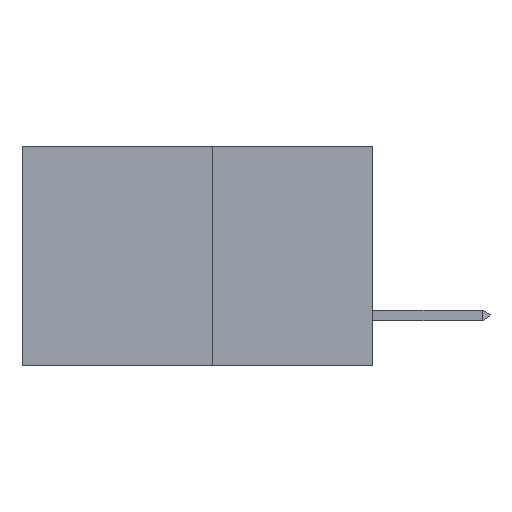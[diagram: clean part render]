
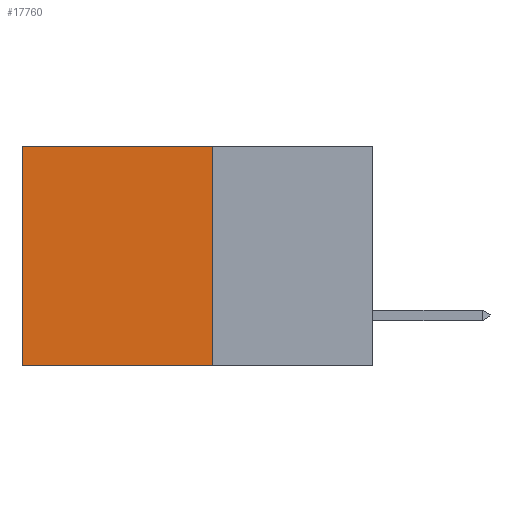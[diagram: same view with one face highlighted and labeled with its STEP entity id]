
A CAD part, left-side view. The second image highlights one B-rep face of the part: STEP entity #17760.
In plain terms, the highlighted planar face has unit normal (-1, 0, 0).
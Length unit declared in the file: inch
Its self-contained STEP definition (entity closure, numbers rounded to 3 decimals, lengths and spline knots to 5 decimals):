
#334 = CARTESIAN_POINT ( 'NONE',  ( 0.277, 0.27, -0.37 ) ) ;
#460 = VERTEX_POINT ( 'NONE', #13434 ) ;
#634 = DIRECTION ( 'NONE',  ( 0., 0., -1. ) ) ;
#1113 = CARTESIAN_POINT ( 'NONE',  ( 0.277, 0.27, 0. ) ) ;
#1631 = PLANE ( 'NONE',  #6819 ) ;
#2547 = VECTOR ( 'NONE', #6142, 39.37008 ) ;
#2607 = VECTOR ( 'NONE', #12795, 39.37008 ) ;
#2858 = CARTESIAN_POINT ( 'NONE',  ( 0.277, 0.59, -0.37 ) ) ;
#2998 = VERTEX_POINT ( 'NONE', #334 ) ;
#3637 = CARTESIAN_POINT ( 'NONE',  ( 0.277, 0.59, 0. ) ) ;
#3745 = EDGE_CURVE ( 'NONE', #14282, #460, #6698, .T. ) ;
#3871 = ORIENTED_EDGE ( 'NONE', *, *, #11626, .F. ) ;
#4233 = ORIENTED_EDGE ( 'NONE', *, *, #17497, .T. ) ;
#5212 = DIRECTION ( 'NONE',  ( 1., 0., 0. ) ) ;
#5300 = VECTOR ( 'NONE', #15342, 39.37008 ) ;
#6118 = VECTOR ( 'NONE', #634, 39.37008 ) ;
#6142 = DIRECTION ( 'NONE',  ( 0., 1., 0. ) ) ;
#6681 = LINE ( 'NONE', #9421, #6118 ) ;
#6698 = LINE ( 'NONE', #2858, #2607 ) ;
#6819 = AXIS2_PLACEMENT_3D ( 'NONE', #14176, #5212, #17722 ) ;
#7753 = LINE ( 'NONE', #15107, #2547 ) ;
#7921 = FACE_OUTER_BOUND ( 'NONE', #13401, .T. ) ;
#8155 = EDGE_CURVE ( 'NONE', #2998, #460, #7753, .T. ) ;
#9421 = CARTESIAN_POINT ( 'NONE',  ( 0.277, 0.27, -0.37 ) ) ;
#9918 = CARTESIAN_POINT ( 'NONE',  ( 0.277, 0.27, 0. ) ) ;
#11232 = ORIENTED_EDGE ( 'NONE', *, *, #3745, .T. ) ;
#11626 = EDGE_CURVE ( 'NONE', #17487, #2998, #6681, .T. ) ;
#12795 = DIRECTION ( 'NONE',  ( 0., 0., -1. ) ) ;
#13401 = EDGE_LOOP ( 'NONE', ( #11232, #13424, #3871, #4233 ) ) ;
#13424 = ORIENTED_EDGE ( 'NONE', *, *, #8155, .F. ) ;
#13434 = CARTESIAN_POINT ( 'NONE',  ( 0.277, 0.59, -0.37 ) ) ;
#14176 = CARTESIAN_POINT ( 'NONE',  ( 0.277, 0.27, -0.37 ) ) ;
#14282 = VERTEX_POINT ( 'NONE', #3637 ) ;
#14311 = LINE ( 'NONE', #1113, #5300 ) ;
#15107 = CARTESIAN_POINT ( 'NONE',  ( 0.277, 0.27, -0.37 ) ) ;
#15342 = DIRECTION ( 'NONE',  ( 0., 1., 0. ) ) ;
#17487 = VERTEX_POINT ( 'NONE', #9918 ) ;
#17497 = EDGE_CURVE ( 'NONE', #17487, #14282, #14311, .T. ) ;
#17722 = DIRECTION ( 'NONE',  ( 0., 0., -1. ) ) ;
#17760 = ADVANCED_FACE ( 'NONE', ( #7921 ), #1631, .F. ) ;
